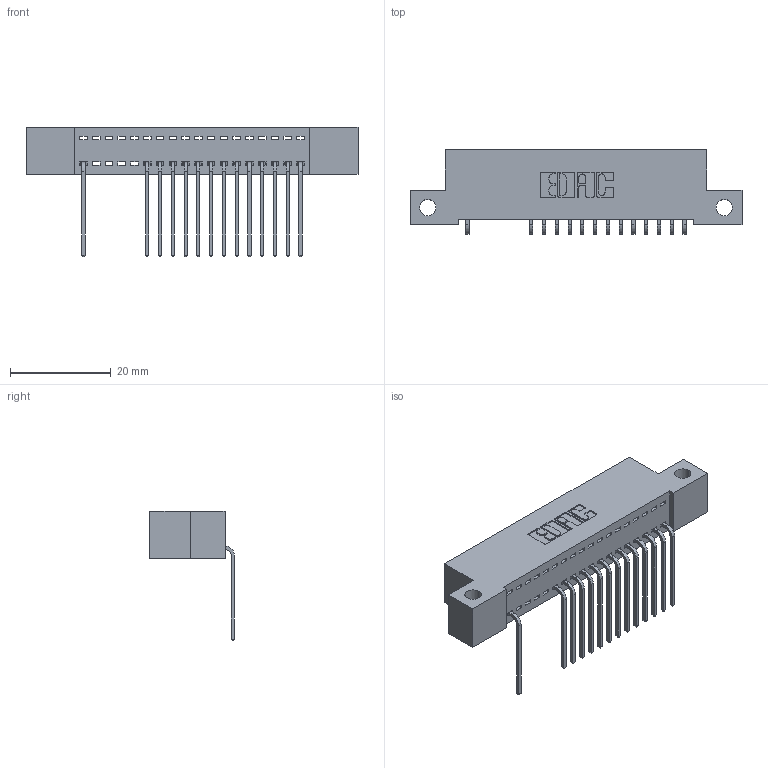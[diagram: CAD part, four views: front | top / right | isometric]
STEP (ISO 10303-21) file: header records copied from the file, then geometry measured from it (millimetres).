
FILE_DESCRIPTION (( 'STEP AP203' ), '1' );
FILE_NAME ('392-018-559-112.STEP', '2018-08-15T04:56:16', ( '' ), ( '' ), 'SwSTEP 2.0', 'SolidWorks 2016', '' );
FILE_SCHEMA (( 'CONFIG_CONTROL_DESIGN' ));
Length unit declared in the file: inch
Products named in the file (3): 342 Part_Side Mount; 345-292-001_558 559 Tail - 1; 392-018-559-112
Assembly tree (15 placements, depth 2):
  392-018-559-112
    342 Part_Side Mount
    345-292-001_558 559 Tail - 1  x14
Bounding box: 66.04 x 16.83 x 25.78 mm (x, y, z)
Volume: 5629 mm3; surface area: 7682.5 mm2
Topology: 15 solids, 15 shells, 998 faces, 3015 edges, 1990 vertices
Faces by surface type: plane 730, cylinder 268
Entity records: 13935 total; most frequent: CARTESIAN_POINT 2432, ORIENTED_EDGE 2390, DIRECTION 2095, EDGE_CURVE 1195, VECTOR 1067, LINE 1067, VERTEX_POINT 794, AXIS2_PLACEMENT_3D 514
